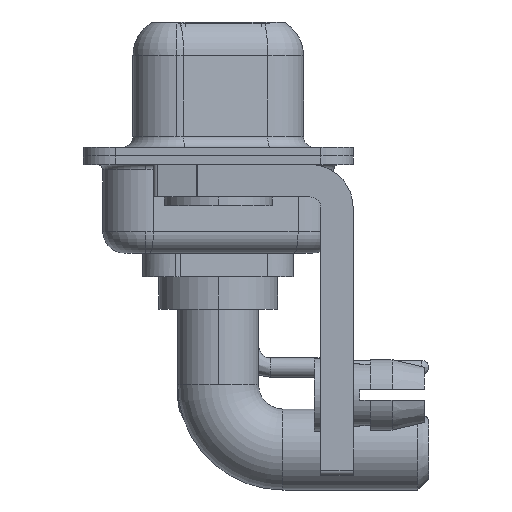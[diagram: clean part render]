
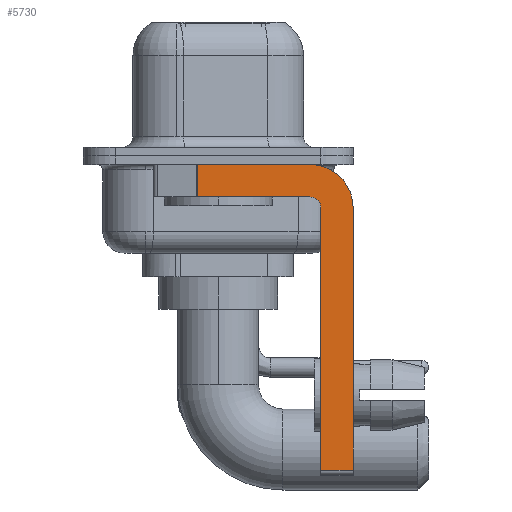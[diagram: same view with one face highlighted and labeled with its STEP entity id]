
A CAD part, left-side view. The second image highlights one B-rep face of the part: STEP entity #5730.
In plain terms, the highlighted planar face has unit normal (-1, 0, 0).
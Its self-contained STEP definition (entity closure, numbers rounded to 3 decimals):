
#98 = AXIS2_PLACEMENT_3D ( 'NONE', #8508, #16362, #8807 ) ;
#144 = VECTOR ( 'NONE', #3715, 1000. ) ;
#301 = CARTESIAN_POINT ( 'NONE',  ( -2.9, -6.25, -14.55 ) ) ;
#629 = EDGE_CURVE ( 'NONE', #2053, #12330, #7430, .T. ) ;
#1165 = DIRECTION ( 'NONE',  ( 1., 0., 0. ) ) ;
#1432 = EDGE_CURVE ( 'NONE', #4860, #14888, #17701, .T. ) ;
#1496 = CARTESIAN_POINT ( 'NONE',  ( -2.9, 0.978, -0.4 ) ) ;
#1499 = LINE ( 'NONE', #7543, #18538 ) ;
#2053 = VERTEX_POINT ( 'NONE', #7419 ) ;
#2217 = EDGE_LOOP ( 'NONE', ( #12776, #19177, #4021, #13418, #14996, #14691, #10827, #19538 ) ) ;
#2411 = CARTESIAN_POINT ( 'NONE',  ( -2.9, -4.25, -0.4 ) ) ;
#3266 = DIRECTION ( 'NONE',  ( 0., -1., 0. ) ) ;
#3539 = LINE ( 'NONE', #10729, #5905 ) ;
#3715 = DIRECTION ( 'NONE',  ( 0., -1., 0. ) ) ;
#3851 = DIRECTION ( 'NONE',  ( 0., 0., 1. ) ) ;
#3941 = VECTOR ( 'NONE', #3851, 1000. ) ;
#4021 = ORIENTED_EDGE ( 'NONE', *, *, #15927, .F. ) ;
#4036 = CARTESIAN_POINT ( 'NONE',  ( -2.9, -4.75, -14.8 ) ) ;
#4860 = VERTEX_POINT ( 'NONE', #9494 ) ;
#5391 = LINE ( 'NONE', #9782, #7768 ) ;
#5722 = DIRECTION ( 'NONE',  ( 0., 0., -1. ) ) ;
#5730 = ADVANCED_FACE ( 'NONE', ( #10013 ), #16073, .F. ) ;
#5757 = EDGE_CURVE ( 'NONE', #12026, #19068, #15981, .T. ) ;
#5832 = CARTESIAN_POINT ( 'NONE',  ( -2.9, 0.978, -1.9 ) ) ;
#5905 = VECTOR ( 'NONE', #9860, 1000. ) ;
#6010 = DIRECTION ( 'NONE',  ( -1., 0., 0. ) ) ;
#6591 = DIRECTION ( 'NONE',  ( 0., 0., -1. ) ) ;
#6742 = EDGE_CURVE ( 'NONE', #10952, #12026, #11270, .T. ) ;
#7419 = CARTESIAN_POINT ( 'NONE',  ( -2.9, -4.75, -14.55 ) ) ;
#7430 = LINE ( 'NONE', #13793, #16403 ) ;
#7543 = CARTESIAN_POINT ( 'NONE',  ( -2.9, -6.25, -2.4 ) ) ;
#7768 = VECTOR ( 'NONE', #6591, 1000. ) ;
#8508 = CARTESIAN_POINT ( 'NONE',  ( -2.9, -4.25, -2.4 ) ) ;
#8807 = DIRECTION ( 'NONE',  ( 0., 0., -1. ) ) ;
#9143 = AXIS2_PLACEMENT_3D ( 'NONE', #14842, #6010, #12075 ) ;
#9494 = CARTESIAN_POINT ( 'NONE',  ( -2.9, -4.75, -2.4 ) ) ;
#9782 = CARTESIAN_POINT ( 'NONE',  ( -2.9, 0.978, -1.9 ) ) ;
#9860 = DIRECTION ( 'NONE',  ( 0., 1., 0. ) ) ;
#9953 = AXIS2_PLACEMENT_3D ( 'NONE', #14754, #1165, #5722 ) ;
#10013 = FACE_OUTER_BOUND ( 'NONE', #2217, .T. ) ;
#10729 = CARTESIAN_POINT ( 'NONE',  ( -2.9, -4.25, -1.9 ) ) ;
#10827 = ORIENTED_EDGE ( 'NONE', *, *, #12249, .F. ) ;
#10952 = VERTEX_POINT ( 'NONE', #1496 ) ;
#11270 = LINE ( 'NONE', #17330, #144 ) ;
#12026 = VERTEX_POINT ( 'NONE', #2411 ) ;
#12031 = DIRECTION ( 'NONE',  ( 0., 0., -1. ) ) ;
#12075 = DIRECTION ( 'NONE',  ( 0., 0., 1. ) ) ;
#12171 = CARTESIAN_POINT ( 'NONE',  ( -2.9, -6.25, -2.4 ) ) ;
#12249 = EDGE_CURVE ( 'NONE', #19068, #12330, #1499, .T. ) ;
#12330 = VERTEX_POINT ( 'NONE', #301 ) ;
#12776 = ORIENTED_EDGE ( 'NONE', *, *, #6742, .F. ) ;
#13418 = ORIENTED_EDGE ( 'NONE', *, *, #1432, .F. ) ;
#13793 = CARTESIAN_POINT ( 'NONE',  ( -2.9, -4.25, -14.55 ) ) ;
#14204 = EDGE_CURVE ( 'NONE', #2053, #4860, #19048, .T. ) ;
#14691 = ORIENTED_EDGE ( 'NONE', *, *, #629, .T. ) ;
#14754 = CARTESIAN_POINT ( 'NONE',  ( -2.9, -4.25, -2.4 ) ) ;
#14842 = CARTESIAN_POINT ( 'NONE',  ( -2.9, -4.25, -2.4 ) ) ;
#14888 = VERTEX_POINT ( 'NONE', #16535 ) ;
#14996 = ORIENTED_EDGE ( 'NONE', *, *, #14204, .F. ) ;
#15198 = EDGE_CURVE ( 'NONE', #10952, #18156, #5391, .T. ) ;
#15927 = EDGE_CURVE ( 'NONE', #14888, #18156, #3539, .T. ) ;
#15981 = CIRCLE ( 'NONE', #98, 2. ) ;
#16073 = PLANE ( 'NONE',  #9953 ) ;
#16362 = DIRECTION ( 'NONE',  ( 1., 0., 0. ) ) ;
#16403 = VECTOR ( 'NONE', #3266, 1000. ) ;
#16535 = CARTESIAN_POINT ( 'NONE',  ( -2.9, -4.25, -1.9 ) ) ;
#17330 = CARTESIAN_POINT ( 'NONE',  ( -2.9, 3., -0.4 ) ) ;
#17701 = CIRCLE ( 'NONE', #9143, 0.5 ) ;
#18156 = VERTEX_POINT ( 'NONE', #5832 ) ;
#18538 = VECTOR ( 'NONE', #12031, 1000. ) ;
#19048 = LINE ( 'NONE', #4036, #3941 ) ;
#19068 = VERTEX_POINT ( 'NONE', #12171 ) ;
#19177 = ORIENTED_EDGE ( 'NONE', *, *, #15198, .T. ) ;
#19538 = ORIENTED_EDGE ( 'NONE', *, *, #5757, .F. ) ;
